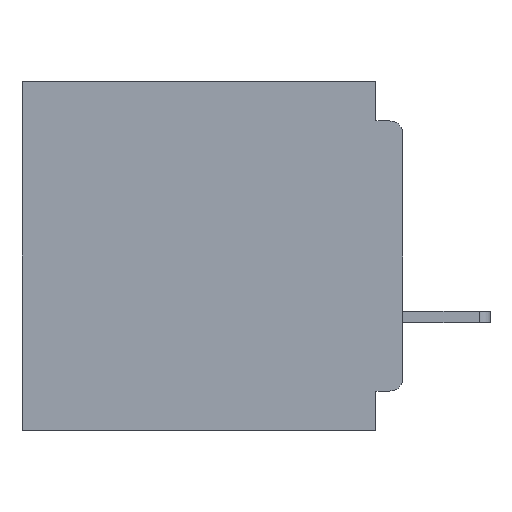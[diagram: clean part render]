
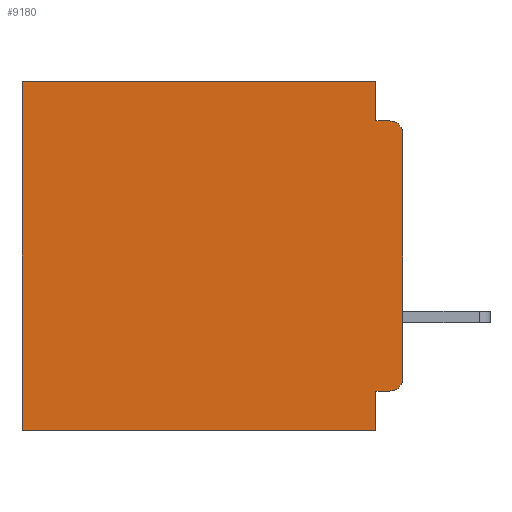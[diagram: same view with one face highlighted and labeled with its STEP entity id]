
A CAD part, left-side view. The second image highlights one B-rep face of the part: STEP entity #9180.
In plain terms, the highlighted planar face has unit normal (-1, 0, 0).
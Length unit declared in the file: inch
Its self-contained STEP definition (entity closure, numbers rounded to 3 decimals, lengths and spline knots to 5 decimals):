
#662 = EDGE_LOOP ( 'NONE', ( #19717, #32913, #52546, #47081, #48635, #54921, #29851, #18206, #34545, #61113 ) ) ;
#1181 = CARTESIAN_POINT ( 'NONE',  ( 0.3, 0.437, -0.4 ) ) ;
#1223 = FACE_OUTER_BOUND ( 'NONE', #662, .T. ) ;
#1389 = AXIS2_PLACEMENT_3D ( 'NONE', #34385, #4404, #39415 ) ;
#1825 = CARTESIAN_POINT ( 'NONE',  ( 0.3, 0.015, -0.355 ) ) ;
#3828 = DIRECTION ( 'NONE',  ( 0., 1., 0. ) ) ;
#4404 = DIRECTION ( 'NONE',  ( -1., 0., 0. ) ) ;
#4470 = EDGE_CURVE ( 'NONE', #53238, #39054, #58383, .T. ) ;
#4697 = CARTESIAN_POINT ( 'NONE',  ( 0.3, 0.437, -0.4 ) ) ;
#8515 = VECTOR ( 'NONE', #33093, 39.37008 ) ;
#9180 = ADVANCED_FACE ( 'NONE', ( #1223 ), #44041, .F. ) ;
#9939 = CARTESIAN_POINT ( 'NONE',  ( 0.3, 0.015, -0.34 ) ) ;
#10090 = LINE ( 'NONE', #42944, #8515 ) ;
#12564 = EDGE_CURVE ( 'NONE', #34190, #59852, #48415, .T. ) ;
#13133 = DIRECTION ( 'NONE',  ( 0., 0., -1. ) ) ;
#14143 = CARTESIAN_POINT ( 'NONE',  ( 0.3, 0., -0.4 ) ) ;
#14531 = CARTESIAN_POINT ( 'NONE',  ( 0.3, 0.031, -0.4 ) ) ;
#15015 = DIRECTION ( 'NONE',  ( 0., 0., -1. ) ) ;
#18159 = EDGE_CURVE ( 'NONE', #29461, #63461, #10090, .T. ) ;
#18206 = ORIENTED_EDGE ( 'NONE', *, *, #20092, .F. ) ;
#19189 = DIRECTION ( 'NONE',  ( 1., 0., 0. ) ) ;
#19717 = ORIENTED_EDGE ( 'NONE', *, *, #18159, .F. ) ;
#20092 = EDGE_CURVE ( 'NONE', #64507, #37319, #20150, .T. ) ;
#20103 = CIRCLE ( 'NONE', #1389, 0.015 ) ;
#20119 = CARTESIAN_POINT ( 'NONE',  ( 0.3, 0., -0.355 ) ) ;
#20150 = LINE ( 'NONE', #37975, #31791 ) ;
#20510 = LINE ( 'NONE', #4697, #33723 ) ;
#22595 = CARTESIAN_POINT ( 'NONE',  ( 0.3, 0.031, 0. ) ) ;
#23714 = EDGE_CURVE ( 'NONE', #32671, #63461, #50089, .T. ) ;
#24111 = LINE ( 'NONE', #33826, #50659 ) ;
#25113 = DIRECTION ( 'NONE',  ( 0., 1., 0. ) ) ;
#25467 = AXIS2_PLACEMENT_3D ( 'NONE', #9939, #44891, #15015 ) ;
#25929 = VERTEX_POINT ( 'NONE', #1181 ) ;
#27745 = CARTESIAN_POINT ( 'NONE',  ( 0.3, 0., -0.34 ) ) ;
#29398 = CARTESIAN_POINT ( 'NONE',  ( 0.3, 0., -0.045 ) ) ;
#29461 = VERTEX_POINT ( 'NONE', #40693 ) ;
#29851 = ORIENTED_EDGE ( 'NONE', *, *, #30935, .F. ) ;
#30587 = VECTOR ( 'NONE', #25113, 39.37008 ) ;
#30935 = EDGE_CURVE ( 'NONE', #37319, #25929, #24111, .T. ) ;
#31683 = EDGE_CURVE ( 'NONE', #29461, #39054, #20103, .T. ) ;
#31791 = VECTOR ( 'NONE', #13133, 39.37008 ) ;
#32671 = VERTEX_POINT ( 'NONE', #1825 ) ;
#32913 = ORIENTED_EDGE ( 'NONE', *, *, #31683, .T. ) ;
#33093 = DIRECTION ( 'NONE',  ( 0., 0., -1. ) ) ;
#33398 = AXIS2_PLACEMENT_3D ( 'NONE', #14143, #19189, #54130 ) ;
#33723 = VECTOR ( 'NONE', #59577, 39.37008 ) ;
#33826 = CARTESIAN_POINT ( 'NONE',  ( 0.3, 0., -0.4 ) ) ;
#34190 = VERTEX_POINT ( 'NONE', #22595 ) ;
#34385 = CARTESIAN_POINT ( 'NONE',  ( 0.3, 0.015, -0.06 ) ) ;
#34545 = ORIENTED_EDGE ( 'NONE', *, *, #41744, .F. ) ;
#36206 = CARTESIAN_POINT ( 'NONE',  ( 0.3, 0.437, 0. ) ) ;
#36550 = EDGE_CURVE ( 'NONE', #34190, #53238, #37810, .T. ) ;
#37319 = VERTEX_POINT ( 'NONE', #14531 ) ;
#37810 = LINE ( 'NONE', #58048, #49611 ) ;
#37975 = CARTESIAN_POINT ( 'NONE',  ( 0.3, 0.031, -0.4 ) ) ;
#38367 = CARTESIAN_POINT ( 'NONE',  ( 0.3, 0., 0. ) ) ;
#39020 = DIRECTION ( 'NONE',  ( 0., -1., 0. ) ) ;
#39054 = VERTEX_POINT ( 'NONE', #60782 ) ;
#39415 = DIRECTION ( 'NONE',  ( 0., 0., -1. ) ) ;
#40693 = CARTESIAN_POINT ( 'NONE',  ( 0.3, 0., -0.06 ) ) ;
#41668 = EDGE_CURVE ( 'NONE', #59852, #25929, #20510, .T. ) ;
#41744 = EDGE_CURVE ( 'NONE', #32671, #64507, #57168, .T. ) ;
#41981 = CARTESIAN_POINT ( 'NONE',  ( 0.3, 0.031, -0.045 ) ) ;
#42944 = CARTESIAN_POINT ( 'NONE',  ( 0.3, 0., -0.4 ) ) ;
#43431 = DIRECTION ( 'NONE',  ( 0., 1., 0. ) ) ;
#43694 = VECTOR ( 'NONE', #43431, 39.37008 ) ;
#44041 = PLANE ( 'NONE',  #33398 ) ;
#44891 = DIRECTION ( 'NONE',  ( -1., 0., 0. ) ) ;
#45711 = CARTESIAN_POINT ( 'NONE',  ( 0.3, 0.031, -0.355 ) ) ;
#47081 = ORIENTED_EDGE ( 'NONE', *, *, #36550, .F. ) ;
#48415 = LINE ( 'NONE', #38367, #43694 ) ;
#48635 = ORIENTED_EDGE ( 'NONE', *, *, #12564, .T. ) ;
#49611 = VECTOR ( 'NONE', #53490, 39.37008 ) ;
#50089 = CIRCLE ( 'NONE', #25467, 0.015 ) ;
#50659 = VECTOR ( 'NONE', #3828, 39.37008 ) ;
#52546 = ORIENTED_EDGE ( 'NONE', *, *, #4470, .F. ) ;
#53238 = VERTEX_POINT ( 'NONE', #41981 ) ;
#53490 = DIRECTION ( 'NONE',  ( 0., 0., -1. ) ) ;
#54130 = DIRECTION ( 'NONE',  ( 0., 0., -1. ) ) ;
#54921 = ORIENTED_EDGE ( 'NONE', *, *, #41668, .T. ) ;
#55299 = VECTOR ( 'NONE', #39020, 39.37008 ) ;
#57168 = LINE ( 'NONE', #20119, #30587 ) ;
#58048 = CARTESIAN_POINT ( 'NONE',  ( 0.3, 0.031, 0. ) ) ;
#58383 = LINE ( 'NONE', #29398, #55299 ) ;
#59577 = DIRECTION ( 'NONE',  ( 0., 0., -1. ) ) ;
#59852 = VERTEX_POINT ( 'NONE', #36206 ) ;
#60782 = CARTESIAN_POINT ( 'NONE',  ( 0.3, 0.015, -0.045 ) ) ;
#61113 = ORIENTED_EDGE ( 'NONE', *, *, #23714, .T. ) ;
#63461 = VERTEX_POINT ( 'NONE', #27745 ) ;
#64507 = VERTEX_POINT ( 'NONE', #45711 ) ;
